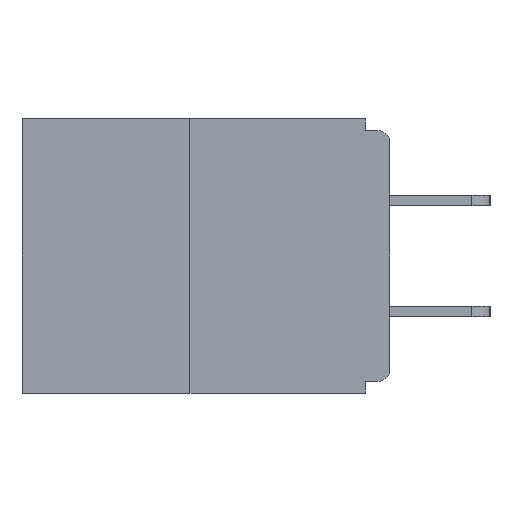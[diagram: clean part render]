
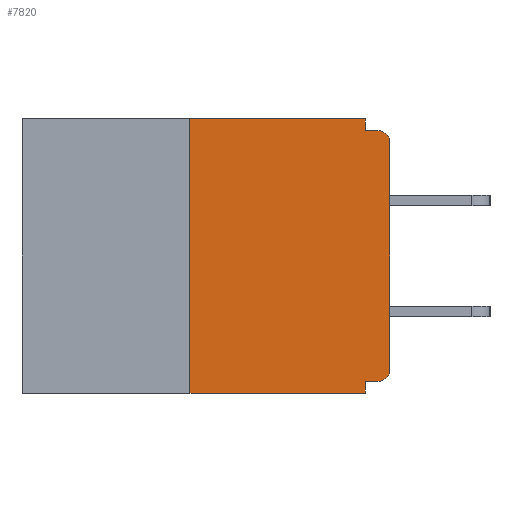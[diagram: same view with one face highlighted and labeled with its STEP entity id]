
A CAD part, left-side view. The second image highlights one B-rep face of the part: STEP entity #7820.
In plain terms, the highlighted planar face has unit normal (-1, 0, 0).
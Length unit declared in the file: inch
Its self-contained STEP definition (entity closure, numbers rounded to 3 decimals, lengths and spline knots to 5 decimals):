
#25 = CARTESIAN_POINT ( 'NONE',  ( 0., 0.015, -0.328 ) ) ;
#87 = LINE ( 'NONE', #211, #6453 ) ;
#211 = CARTESIAN_POINT ( 'NONE',  ( 0., 0.031, -0.343 ) ) ;
#503 = DIRECTION ( 'NONE',  ( 0., -1., 0. ) ) ;
#646 = CIRCLE ( 'NONE', #7523, 0.015 ) ;
#648 = CARTESIAN_POINT ( 'NONE',  ( 0., 0., -0.03 ) ) ;
#658 = DIRECTION ( 'NONE',  ( 0., 0., 1. ) ) ;
#924 = DIRECTION ( 'NONE',  ( 1., 0., 0. ) ) ;
#1537 = EDGE_CURVE ( 'NONE', #1666, #6800, #87, .T. ) ;
#1643 = VERTEX_POINT ( 'NONE', #5513 ) ;
#1666 = VERTEX_POINT ( 'NONE', #10893 ) ;
#1760 = EDGE_CURVE ( 'NONE', #6165, #1666, #3142, .T. ) ;
#1875 = CARTESIAN_POINT ( 'NONE',  ( 0., 0.015, -0.313 ) ) ;
#2133 = CARTESIAN_POINT ( 'NONE',  ( 0., 0.46, 0. ) ) ;
#2394 = VERTEX_POINT ( 'NONE', #2852 ) ;
#2442 = DIRECTION ( 'NONE',  ( 0., -1., 0. ) ) ;
#2467 = PLANE ( 'NONE',  #5136 ) ;
#2497 = VERTEX_POINT ( 'NONE', #4473 ) ;
#2506 = CARTESIAN_POINT ( 'NONE',  ( 0., 0., -0.015 ) ) ;
#2597 = LINE ( 'NONE', #4156, #6967 ) ;
#2749 = ORIENTED_EDGE ( 'NONE', *, *, #9648, .T. ) ;
#2852 = CARTESIAN_POINT ( 'NONE',  ( 0., 0.031, 0. ) ) ;
#3006 = VERTEX_POINT ( 'NONE', #648 ) ;
#3052 = VERTEX_POINT ( 'NONE', #9257 ) ;
#3142 = LINE ( 'NONE', #7502, #8279 ) ;
#3148 = EDGE_CURVE ( 'NONE', #3006, #9106, #6769, .T. ) ;
#3154 = DIRECTION ( 'NONE',  ( 0., 0., -1. ) ) ;
#3308 = EDGE_CURVE ( 'NONE', #3052, #2394, #8174, .T. ) ;
#3364 = CARTESIAN_POINT ( 'NONE',  ( 0., 0.015, -0.03 ) ) ;
#3394 = ORIENTED_EDGE ( 'NONE', *, *, #9800, .T. ) ;
#3619 = DIRECTION ( 'NONE',  ( 0., 0., -1. ) ) ;
#3773 = DIRECTION ( 'NONE',  ( 0., 0., -1. ) ) ;
#3793 = ORIENTED_EDGE ( 'NONE', *, *, #9488, .F. ) ;
#4156 = CARTESIAN_POINT ( 'NONE',  ( 0., 0., 0. ) ) ;
#4252 = VECTOR ( 'NONE', #503, 39.37008 ) ;
#4308 = FACE_OUTER_BOUND ( 'NONE', #4614, .T. ) ;
#4430 = VECTOR ( 'NONE', #2442, 39.37008 ) ;
#4448 = ORIENTED_EDGE ( 'NONE', *, *, #3308, .F. ) ;
#4473 = CARTESIAN_POINT ( 'NONE',  ( 0., 0.031, -0.015 ) ) ;
#4614 = EDGE_LOOP ( 'NONE', ( #4448, #9330, #3394, #7141, #6182, #2749, #8050, #5814, #3793, #8734 ) ) ;
#4850 = DIRECTION ( 'NONE',  ( 0., 1., 0. ) ) ;
#4867 = LINE ( 'NONE', #8992, #4252 ) ;
#5136 = AXIS2_PLACEMENT_3D ( 'NONE', #7784, #924, #10364 ) ;
#5453 = CARTESIAN_POINT ( 'NONE',  ( 0., 0.015, -0.015 ) ) ;
#5513 = CARTESIAN_POINT ( 'NONE',  ( 0., 0., -0.313 ) ) ;
#5617 = DIRECTION ( 'NONE',  ( 0., -1., 0. ) ) ;
#5814 = ORIENTED_EDGE ( 'NONE', *, *, #3148, .T. ) ;
#6059 = AXIS2_PLACEMENT_3D ( 'NONE', #3364, #11183, #6811 ) ;
#6165 = VERTEX_POINT ( 'NONE', #25 ) ;
#6182 = ORIENTED_EDGE ( 'NONE', *, *, #1760, .F. ) ;
#6227 = LINE ( 'NONE', #10472, #9178 ) ;
#6453 = VECTOR ( 'NONE', #3773, 39.37008 ) ;
#6516 = CARTESIAN_POINT ( 'NONE',  ( 0., 0.031, -0.343 ) ) ;
#6769 = CIRCLE ( 'NONE', #6059, 0.015 ) ;
#6800 = VERTEX_POINT ( 'NONE', #6516 ) ;
#6811 = DIRECTION ( 'NONE',  ( 0., 0., -1. ) ) ;
#6967 = VECTOR ( 'NONE', #658, 39.37008 ) ;
#7044 = EDGE_CURVE ( 'NONE', #10823, #3052, #6227, .T. ) ;
#7141 = ORIENTED_EDGE ( 'NONE', *, *, #1537, .F. ) ;
#7352 = LINE ( 'NONE', #9215, #9501 ) ;
#7502 = CARTESIAN_POINT ( 'NONE',  ( 0., 0., -0.328 ) ) ;
#7523 = AXIS2_PLACEMENT_3D ( 'NONE', #1875, #8712, #3619 ) ;
#7691 = VECTOR ( 'NONE', #5617, 39.37008 ) ;
#7784 = CARTESIAN_POINT ( 'NONE',  ( 0., 0.46, 0. ) ) ;
#7820 = ADVANCED_FACE ( 'NONE', ( #4308 ), #2467, .F. ) ;
#7937 = DIRECTION ( 'NONE',  ( 0., 0., 1. ) ) ;
#8050 = ORIENTED_EDGE ( 'NONE', *, *, #9946, .T. ) ;
#8174 = LINE ( 'NONE', #2133, #7691 ) ;
#8279 = VECTOR ( 'NONE', #4850, 39.37008 ) ;
#8712 = DIRECTION ( 'NONE',  ( -1., 0., 0. ) ) ;
#8734 = ORIENTED_EDGE ( 'NONE', *, *, #9722, .F. ) ;
#8992 = CARTESIAN_POINT ( 'NONE',  ( 0., 0.46, -0.343 ) ) ;
#9106 = VERTEX_POINT ( 'NONE', #5453 ) ;
#9178 = VECTOR ( 'NONE', #7937, 39.37008 ) ;
#9215 = CARTESIAN_POINT ( 'NONE',  ( 0., 0.031, 0. ) ) ;
#9257 = CARTESIAN_POINT ( 'NONE',  ( 0., 0.25, 0. ) ) ;
#9330 = ORIENTED_EDGE ( 'NONE', *, *, #7044, .F. ) ;
#9488 = EDGE_CURVE ( 'NONE', #2497, #9106, #11074, .T. ) ;
#9501 = VECTOR ( 'NONE', #3154, 39.37008 ) ;
#9648 = EDGE_CURVE ( 'NONE', #6165, #1643, #646, .T. ) ;
#9722 = EDGE_CURVE ( 'NONE', #2394, #2497, #7352, .T. ) ;
#9800 = EDGE_CURVE ( 'NONE', #10823, #6800, #4867, .T. ) ;
#9946 = EDGE_CURVE ( 'NONE', #1643, #3006, #2597, .T. ) ;
#10364 = DIRECTION ( 'NONE',  ( 0., 0., -1. ) ) ;
#10472 = CARTESIAN_POINT ( 'NONE',  ( 0., 0.25, 0. ) ) ;
#10823 = VERTEX_POINT ( 'NONE', #11160 ) ;
#10893 = CARTESIAN_POINT ( 'NONE',  ( 0., 0.031, -0.328 ) ) ;
#11074 = LINE ( 'NONE', #2506, #4430 ) ;
#11160 = CARTESIAN_POINT ( 'NONE',  ( 0., 0.25, -0.343 ) ) ;
#11183 = DIRECTION ( 'NONE',  ( -1., 0., 0. ) ) ;
